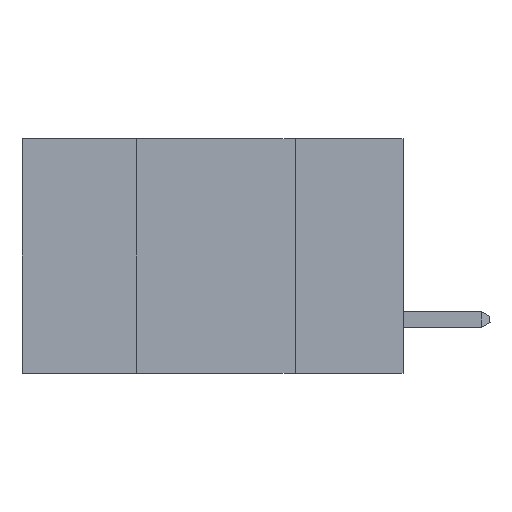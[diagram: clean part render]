
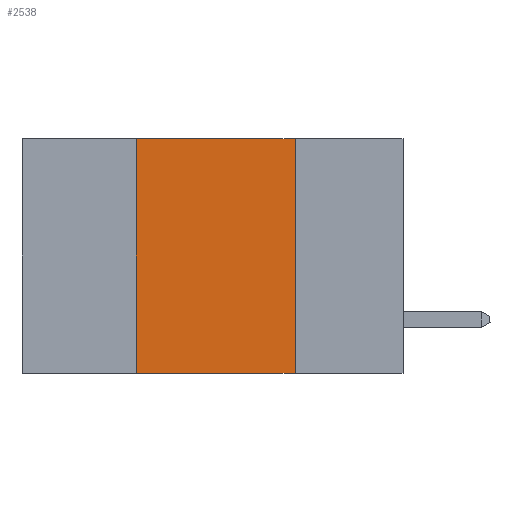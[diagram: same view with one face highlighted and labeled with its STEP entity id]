
A CAD part, left-side view. The second image highlights one B-rep face of the part: STEP entity #2538.
In plain terms, the highlighted planar face has unit normal (-1, 0, 0).
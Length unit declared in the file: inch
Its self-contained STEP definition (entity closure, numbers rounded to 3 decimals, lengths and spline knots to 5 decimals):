
#17 = VERTEX_POINT ( 'NONE', #5089 ) ;
#41 = VECTOR ( 'NONE', #2130, 39.37008 ) ;
#484 = CARTESIAN_POINT ( 'NONE',  ( 0., 0.17, 0. ) ) ;
#619 = DIRECTION ( 'NONE',  ( 0., -1., 0. ) ) ;
#776 = DIRECTION ( 'NONE',  ( 0., 0., 1. ) ) ;
#1188 = ORIENTED_EDGE ( 'NONE', *, *, #9925, .T. ) ;
#1378 = CARTESIAN_POINT ( 'NONE',  ( 0., 0.42, 0. ) ) ;
#1460 = FACE_OUTER_BOUND ( 'NONE', #4101, .T. ) ;
#2064 = EDGE_CURVE ( 'NONE', #17, #10366, #3293, .T. ) ;
#2130 = DIRECTION ( 'NONE',  ( 0., -1., 0. ) ) ;
#2173 = CARTESIAN_POINT ( 'NONE',  ( 0., 0.6, 0. ) ) ;
#2240 = PLANE ( 'NONE',  #2647 ) ;
#2490 = EDGE_CURVE ( 'NONE', #10366, #10421, #5589, .T. ) ;
#2538 = ADVANCED_FACE ( 'NONE', ( #1460 ), #2240, .F. ) ;
#2647 = AXIS2_PLACEMENT_3D ( 'NONE', #2173, #7991, #8864 ) ;
#3012 = DIRECTION ( 'NONE',  ( 0., 0., -1. ) ) ;
#3111 = CARTESIAN_POINT ( 'NONE',  ( 0., 0.42, 0. ) ) ;
#3122 = CARTESIAN_POINT ( 'NONE',  ( 0., 0.17, -0.37 ) ) ;
#3293 = LINE ( 'NONE', #1378, #8903 ) ;
#3484 = VERTEX_POINT ( 'NONE', #3122 ) ;
#3757 = CARTESIAN_POINT ( 'NONE',  ( 0., 0.6, 0. ) ) ;
#4101 = EDGE_LOOP ( 'NONE', ( #4411, #7182, #7943, #1188 ) ) ;
#4411 = ORIENTED_EDGE ( 'NONE', *, *, #5396, .F. ) ;
#5089 = CARTESIAN_POINT ( 'NONE',  ( 0., 0.42, -0.37 ) ) ;
#5396 = EDGE_CURVE ( 'NONE', #10421, #3484, #8039, .T. ) ;
#5481 = CARTESIAN_POINT ( 'NONE',  ( 0., 0.6, -0.37 ) ) ;
#5589 = LINE ( 'NONE', #3757, #10702 ) ;
#7182 = ORIENTED_EDGE ( 'NONE', *, *, #2490, .F. ) ;
#7743 = CARTESIAN_POINT ( 'NONE',  ( 0., 0.17, 0. ) ) ;
#7861 = LINE ( 'NONE', #5481, #41 ) ;
#7943 = ORIENTED_EDGE ( 'NONE', *, *, #2064, .F. ) ;
#7991 = DIRECTION ( 'NONE',  ( 1., 0., 0. ) ) ;
#8039 = LINE ( 'NONE', #484, #9612 ) ;
#8864 = DIRECTION ( 'NONE',  ( 0., 0., -1. ) ) ;
#8903 = VECTOR ( 'NONE', #776, 39.37008 ) ;
#9612 = VECTOR ( 'NONE', #3012, 39.37008 ) ;
#9925 = EDGE_CURVE ( 'NONE', #17, #3484, #7861, .T. ) ;
#10366 = VERTEX_POINT ( 'NONE', #3111 ) ;
#10421 = VERTEX_POINT ( 'NONE', #7743 ) ;
#10702 = VECTOR ( 'NONE', #619, 39.37008 ) ;
